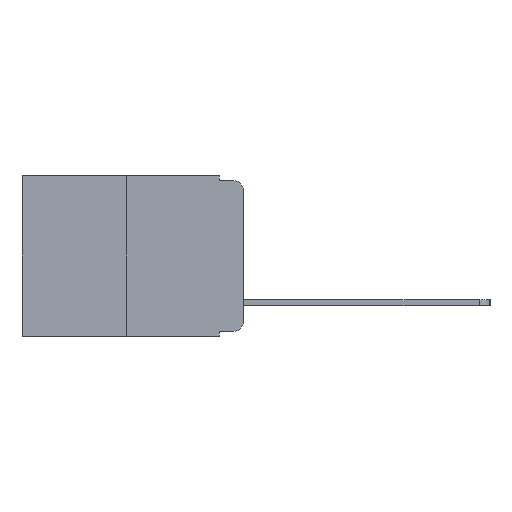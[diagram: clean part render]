
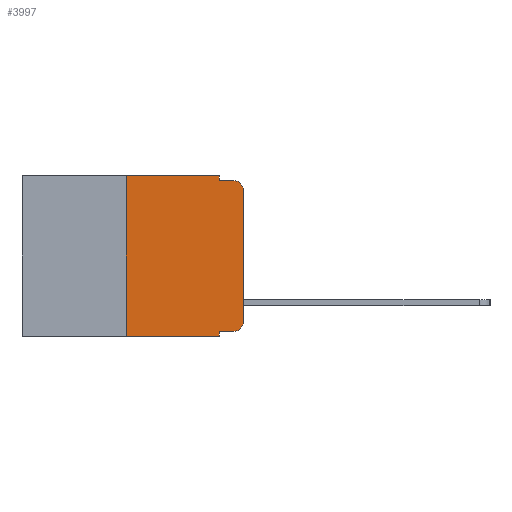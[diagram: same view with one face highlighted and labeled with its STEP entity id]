
A CAD part, left-side view. The second image highlights one B-rep face of the part: STEP entity #3997.
In plain terms, the highlighted planar face has unit normal (-1, 0, 0).
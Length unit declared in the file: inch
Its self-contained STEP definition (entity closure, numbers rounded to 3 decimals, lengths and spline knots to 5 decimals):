
#58 = VERTEX_POINT ( 'NONE', #19172 ) ;
#99 = CARTESIAN_POINT ( 'NONE',  ( 0., 0.051, -0.333 ) ) ;
#249 = CIRCLE ( 'NONE', #18780, 0.02 ) ;
#336 = CARTESIAN_POINT ( 'NONE',  ( 0., 0.051, 0. ) ) ;
#619 = CIRCLE ( 'NONE', #6660, 0.02 ) ;
#742 = DIRECTION ( 'NONE',  ( 0., 0., -1. ) ) ;
#752 = ORIENTED_EDGE ( 'NONE', *, *, #6266, .F. ) ;
#785 = LINE ( 'NONE', #6961, #13114 ) ;
#1216 = VERTEX_POINT ( 'NONE', #336 ) ;
#1858 = EDGE_CURVE ( 'NONE', #8729, #58, #249, .T. ) ;
#1874 = CARTESIAN_POINT ( 'NONE',  ( 0., 0.02, -0.01 ) ) ;
#2674 = EDGE_CURVE ( 'NONE', #3617, #15720, #13968, .T. ) ;
#3251 = CARTESIAN_POINT ( 'NONE',  ( 0., 0.051, -0.01 ) ) ;
#3409 = CARTESIAN_POINT ( 'NONE',  ( 0., 0.25, 0. ) ) ;
#3617 = VERTEX_POINT ( 'NONE', #16899 ) ;
#3997 = ADVANCED_FACE ( 'NONE', ( #9724 ), #16203, .F. ) ;
#4171 = EDGE_CURVE ( 'NONE', #1216, #12270, #18130, .T. ) ;
#5047 = DIRECTION ( 'NONE',  ( 0., -1., 0. ) ) ;
#5260 = VERTEX_POINT ( 'NONE', #1874 ) ;
#5576 = ORIENTED_EDGE ( 'NONE', *, *, #5865, .T. ) ;
#5582 = DIRECTION ( 'NONE',  ( 0., -1., 0. ) ) ;
#5865 = EDGE_CURVE ( 'NONE', #14308, #15720, #785, .T. ) ;
#6044 = VECTOR ( 'NONE', #742, 39.37008 ) ;
#6072 = LINE ( 'NONE', #14505, #6533 ) ;
#6266 = EDGE_CURVE ( 'NONE', #14308, #14248, #8200, .T. ) ;
#6269 = CARTESIAN_POINT ( 'NONE',  ( 0., 0., -0.03 ) ) ;
#6502 = CARTESIAN_POINT ( 'NONE',  ( 0., 0.02, -0.03 ) ) ;
#6533 = VECTOR ( 'NONE', #5582, 39.37008 ) ;
#6660 = AXIS2_PLACEMENT_3D ( 'NONE', #6502, #16836, #8035 ) ;
#6961 = CARTESIAN_POINT ( 'NONE',  ( 0., 0.473, -0.343 ) ) ;
#7002 = ORIENTED_EDGE ( 'NONE', *, *, #10342, .T. ) ;
#7122 = CARTESIAN_POINT ( 'NONE',  ( 0., 0.051, -0.343 ) ) ;
#7365 = CARTESIAN_POINT ( 'NONE',  ( 0., 0.02, -0.313 ) ) ;
#7461 = CARTESIAN_POINT ( 'NONE',  ( 0., 0., 0. ) ) ;
#8035 = DIRECTION ( 'NONE',  ( 0., 0., -1. ) ) ;
#8200 = LINE ( 'NONE', #3409, #8696 ) ;
#8597 = CARTESIAN_POINT ( 'NONE',  ( 0., 0.02, -0.333 ) ) ;
#8696 = VECTOR ( 'NONE', #11134, 39.37008 ) ;
#8718 = EDGE_CURVE ( 'NONE', #14248, #1216, #6072, .T. ) ;
#8729 = VERTEX_POINT ( 'NONE', #8597 ) ;
#8827 = DIRECTION ( 'NONE',  ( -1., 0., 0. ) ) ;
#9600 = EDGE_CURVE ( 'NONE', #12270, #5260, #18896, .T. ) ;
#9724 = FACE_OUTER_BOUND ( 'NONE', #12345, .T. ) ;
#9858 = ORIENTED_EDGE ( 'NONE', *, *, #15549, .T. ) ;
#9940 = VECTOR ( 'NONE', #17273, 39.37008 ) ;
#10342 = EDGE_CURVE ( 'NONE', #3617, #8729, #11884, .T. ) ;
#11134 = DIRECTION ( 'NONE',  ( 0., 0., 1. ) ) ;
#11500 = ORIENTED_EDGE ( 'NONE', *, *, #1858, .T. ) ;
#11684 = VECTOR ( 'NONE', #13465, 39.37008 ) ;
#11884 = LINE ( 'NONE', #99, #14813 ) ;
#12034 = CARTESIAN_POINT ( 'NONE',  ( 0., 0.25, 0. ) ) ;
#12156 = LINE ( 'NONE', #7461, #11684 ) ;
#12226 = VERTEX_POINT ( 'NONE', #6269 ) ;
#12270 = VERTEX_POINT ( 'NONE', #18179 ) ;
#12275 = DIRECTION ( 'NONE',  ( 0., 0., -1. ) ) ;
#12345 = EDGE_LOOP ( 'NONE', ( #9858, #18048, #15547, #19389, #16460, #752, #5576, #18275, #7002, #11500 ) ) ;
#12981 = DIRECTION ( 'NONE',  ( 0., -1., 0. ) ) ;
#13114 = VECTOR ( 'NONE', #12981, 39.37008 ) ;
#13364 = CARTESIAN_POINT ( 'NONE',  ( 0., 0.051, 0. ) ) ;
#13465 = DIRECTION ( 'NONE',  ( 0., 0., 1. ) ) ;
#13968 = LINE ( 'NONE', #13364, #6044 ) ;
#14248 = VERTEX_POINT ( 'NONE', #12034 ) ;
#14308 = VERTEX_POINT ( 'NONE', #15063 ) ;
#14505 = CARTESIAN_POINT ( 'NONE',  ( 0., 0.473, 0. ) ) ;
#14813 = VECTOR ( 'NONE', #5047, 39.37008 ) ;
#15063 = CARTESIAN_POINT ( 'NONE',  ( 0., 0.25, -0.343 ) ) ;
#15077 = VECTOR ( 'NONE', #16732, 39.37008 ) ;
#15547 = ORIENTED_EDGE ( 'NONE', *, *, #9600, .F. ) ;
#15549 = EDGE_CURVE ( 'NONE', #58, #12226, #12156, .T. ) ;
#15720 = VERTEX_POINT ( 'NONE', #7122 ) ;
#16165 = CARTESIAN_POINT ( 'NONE',  ( 0., 0.473, 0. ) ) ;
#16203 = PLANE ( 'NONE',  #18112 ) ;
#16460 = ORIENTED_EDGE ( 'NONE', *, *, #8718, .F. ) ;
#16697 = DIRECTION ( 'NONE',  ( 1., 0., 0. ) ) ;
#16732 = DIRECTION ( 'NONE',  ( 0., -1., 0. ) ) ;
#16836 = DIRECTION ( 'NONE',  ( -1., 0., 0. ) ) ;
#16899 = CARTESIAN_POINT ( 'NONE',  ( 0., 0.051, -0.333 ) ) ;
#17121 = DIRECTION ( 'NONE',  ( 0., 0., -1. ) ) ;
#17273 = DIRECTION ( 'NONE',  ( 0., 0., -1. ) ) ;
#18048 = ORIENTED_EDGE ( 'NONE', *, *, #18473, .T. ) ;
#18112 = AXIS2_PLACEMENT_3D ( 'NONE', #16165, #16697, #17121 ) ;
#18130 = LINE ( 'NONE', #18772, #9940 ) ;
#18179 = CARTESIAN_POINT ( 'NONE',  ( 0., 0.051, -0.01 ) ) ;
#18275 = ORIENTED_EDGE ( 'NONE', *, *, #2674, .F. ) ;
#18473 = EDGE_CURVE ( 'NONE', #12226, #5260, #619, .T. ) ;
#18772 = CARTESIAN_POINT ( 'NONE',  ( 0., 0.051, 0. ) ) ;
#18780 = AXIS2_PLACEMENT_3D ( 'NONE', #7365, #8827, #12275 ) ;
#18896 = LINE ( 'NONE', #3251, #15077 ) ;
#19172 = CARTESIAN_POINT ( 'NONE',  ( 0., 0., -0.313 ) ) ;
#19389 = ORIENTED_EDGE ( 'NONE', *, *, #4171, .F. ) ;
